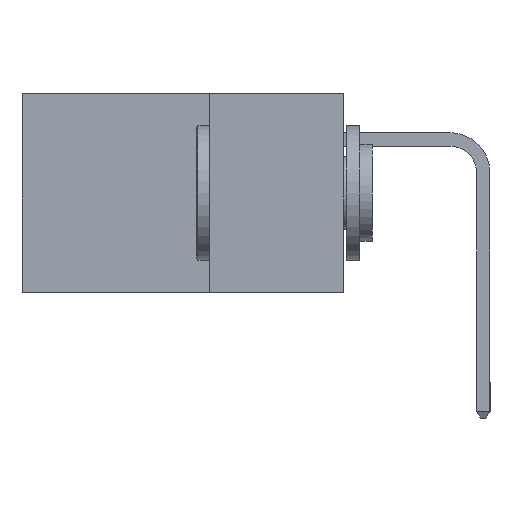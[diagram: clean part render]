
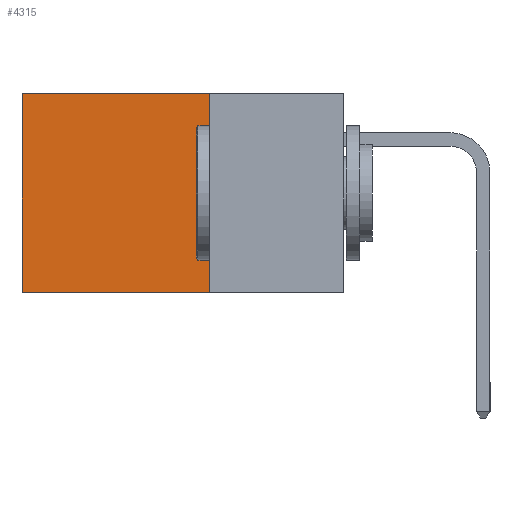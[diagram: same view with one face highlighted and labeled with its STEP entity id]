
A CAD part, left-side view. The second image highlights one B-rep face of the part: STEP entity #4315.
In plain terms, the highlighted planar face has unit normal (-1, 0, 0).
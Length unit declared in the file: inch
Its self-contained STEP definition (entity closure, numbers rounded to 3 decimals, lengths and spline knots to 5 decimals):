
#63 = EDGE_CURVE ( 'NONE', #20325, #11239, #29530, .T. ) ;
#1310 = VECTOR ( 'NONE', #7493, 39.37008 ) ;
#2341 = CARTESIAN_POINT ( 'NONE',  ( 0.298, 0.25, -0.37 ) ) ;
#3281 = VERTEX_POINT ( 'NONE', #4706 ) ;
#3422 = ORIENTED_EDGE ( 'NONE', *, *, #10078, .T. ) ;
#3773 = CARTESIAN_POINT ( 'NONE',  ( 0.298, 0.6, 0. ) ) ;
#4315 = ADVANCED_FACE ( 'NONE', ( #11853 ), #26897, .F. ) ;
#4706 = CARTESIAN_POINT ( 'NONE',  ( 0.298, 0.25, 0. ) ) ;
#6253 = DIRECTION ( 'NONE',  ( 0., 0., -1. ) ) ;
#7493 = DIRECTION ( 'NONE',  ( 0., 0., -1. ) ) ;
#10078 = EDGE_CURVE ( 'NONE', #12846, #11239, #25407, .T. ) ;
#11239 = VERTEX_POINT ( 'NONE', #19079 ) ;
#11513 = DIRECTION ( 'NONE',  ( 0., 1., 0. ) ) ;
#11559 = CARTESIAN_POINT ( 'NONE',  ( 0.298, 0.25, -0.37 ) ) ;
#11827 = CARTESIAN_POINT ( 'NONE',  ( 0.298, 0.25, 0. ) ) ;
#11853 = FACE_OUTER_BOUND ( 'NONE', #29972, .T. ) ;
#12846 = VERTEX_POINT ( 'NONE', #3773 ) ;
#13444 = LINE ( 'NONE', #24875, #19678 ) ;
#16044 = ORIENTED_EDGE ( 'NONE', *, *, #17107, .T. ) ;
#16660 = VECTOR ( 'NONE', #11513, 39.37008 ) ;
#17107 = EDGE_CURVE ( 'NONE', #3281, #12846, #28869, .T. ) ;
#17866 = AXIS2_PLACEMENT_3D ( 'NONE', #11827, #20823, #21688 ) ;
#19079 = CARTESIAN_POINT ( 'NONE',  ( 0.298, 0.6, -0.37 ) ) ;
#19678 = VECTOR ( 'NONE', #6253, 39.37008 ) ;
#20325 = VERTEX_POINT ( 'NONE', #11559 ) ;
#20593 = DIRECTION ( 'NONE',  ( 0., 1., 0. ) ) ;
#20823 = DIRECTION ( 'NONE',  ( 1., 0., 0. ) ) ;
#21688 = DIRECTION ( 'NONE',  ( 0., 0., -1. ) ) ;
#23177 = CARTESIAN_POINT ( 'NONE',  ( 0.298, 0.25, 0. ) ) ;
#23541 = VECTOR ( 'NONE', #20593, 39.37008 ) ;
#24404 = ORIENTED_EDGE ( 'NONE', *, *, #63, .F. ) ;
#24875 = CARTESIAN_POINT ( 'NONE',  ( 0.298, 0.25, 0. ) ) ;
#25407 = LINE ( 'NONE', #26050, #1310 ) ;
#26050 = CARTESIAN_POINT ( 'NONE',  ( 0.298, 0.6, 0. ) ) ;
#26304 = ORIENTED_EDGE ( 'NONE', *, *, #26737, .F. ) ;
#26737 = EDGE_CURVE ( 'NONE', #3281, #20325, #13444, .T. ) ;
#26897 = PLANE ( 'NONE',  #17866 ) ;
#28869 = LINE ( 'NONE', #23177, #16660 ) ;
#29530 = LINE ( 'NONE', #2341, #23541 ) ;
#29972 = EDGE_LOOP ( 'NONE', ( #3422, #24404, #26304, #16044 ) ) ;
